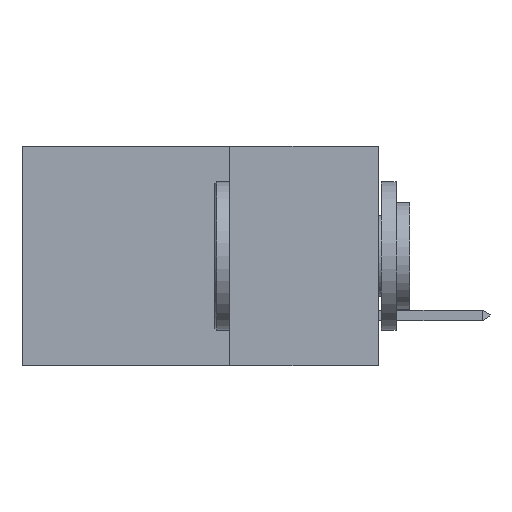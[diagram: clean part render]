
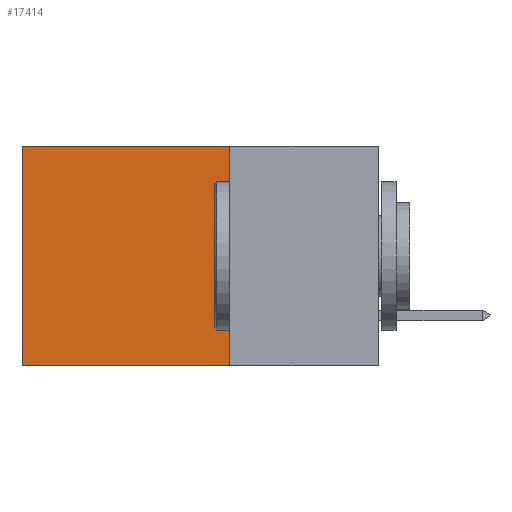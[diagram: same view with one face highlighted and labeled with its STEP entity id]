
A CAD part, left-side view. The second image highlights one B-rep face of the part: STEP entity #17414.
In plain terms, the highlighted planar face has unit normal (-1, 0, 0).
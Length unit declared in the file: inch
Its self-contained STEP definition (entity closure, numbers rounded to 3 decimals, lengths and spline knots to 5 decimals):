
#1201 = DIRECTION ( 'NONE',  ( 0., 1., 0. ) ) ;
#1425 = CARTESIAN_POINT ( 'NONE',  ( 0.298, 0.6, 0. ) ) ;
#2427 = CARTESIAN_POINT ( 'NONE',  ( 0.298, 0.25, -0.37 ) ) ;
#2792 = LINE ( 'NONE', #12776, #9463 ) ;
#2874 = ORIENTED_EDGE ( 'NONE', *, *, #17186, .T. ) ;
#3577 = VECTOR ( 'NONE', #7123, 39.37008 ) ;
#5601 = VERTEX_POINT ( 'NONE', #20308 ) ;
#6472 = CARTESIAN_POINT ( 'NONE',  ( 0.298, 0.25, 0. ) ) ;
#6558 = PLANE ( 'NONE',  #13876 ) ;
#7015 = VERTEX_POINT ( 'NONE', #2427 ) ;
#7123 = DIRECTION ( 'NONE',  ( 0., 0., -1. ) ) ;
#8605 = DIRECTION ( 'NONE',  ( 0., 0., -1. ) ) ;
#9299 = EDGE_CURVE ( 'NONE', #7015, #16319, #19780, .T. ) ;
#9463 = VECTOR ( 'NONE', #17250, 39.37008 ) ;
#9981 = ORIENTED_EDGE ( 'NONE', *, *, #9299, .F. ) ;
#10788 = ORIENTED_EDGE ( 'NONE', *, *, #15073, .F. ) ;
#12470 = LINE ( 'NONE', #19360, #3577 ) ;
#12776 = CARTESIAN_POINT ( 'NONE',  ( 0.298, 0.25, 0. ) ) ;
#13371 = CARTESIAN_POINT ( 'NONE',  ( 0.298, 0.6, 0. ) ) ;
#13592 = CARTESIAN_POINT ( 'NONE',  ( 0.298, 0.25, -0.37 ) ) ;
#13876 = AXIS2_PLACEMENT_3D ( 'NONE', #6472, #16507, #8605 ) ;
#13891 = EDGE_CURVE ( 'NONE', #25619, #16319, #14752, .T. ) ;
#14413 = VECTOR ( 'NONE', #1201, 39.37008 ) ;
#14752 = LINE ( 'NONE', #1425, #22385 ) ;
#15073 = EDGE_CURVE ( 'NONE', #5601, #7015, #12470, .T. ) ;
#15444 = EDGE_LOOP ( 'NONE', ( #22502, #9981, #10788, #2874 ) ) ;
#16319 = VERTEX_POINT ( 'NONE', #20893 ) ;
#16507 = DIRECTION ( 'NONE',  ( 1., 0., 0. ) ) ;
#17186 = EDGE_CURVE ( 'NONE', #5601, #25619, #2792, .T. ) ;
#17250 = DIRECTION ( 'NONE',  ( 0., 1., 0. ) ) ;
#17414 = ADVANCED_FACE ( 'NONE', ( #18682 ), #6558, .F. ) ;
#18682 = FACE_OUTER_BOUND ( 'NONE', #15444, .T. ) ;
#19360 = CARTESIAN_POINT ( 'NONE',  ( 0.298, 0.25, 0. ) ) ;
#19780 = LINE ( 'NONE', #13592, #14413 ) ;
#19826 = DIRECTION ( 'NONE',  ( 0., 0., -1. ) ) ;
#20308 = CARTESIAN_POINT ( 'NONE',  ( 0.298, 0.25, 0. ) ) ;
#20893 = CARTESIAN_POINT ( 'NONE',  ( 0.298, 0.6, -0.37 ) ) ;
#22385 = VECTOR ( 'NONE', #19826, 39.37008 ) ;
#22502 = ORIENTED_EDGE ( 'NONE', *, *, #13891, .T. ) ;
#25619 = VERTEX_POINT ( 'NONE', #13371 ) ;
